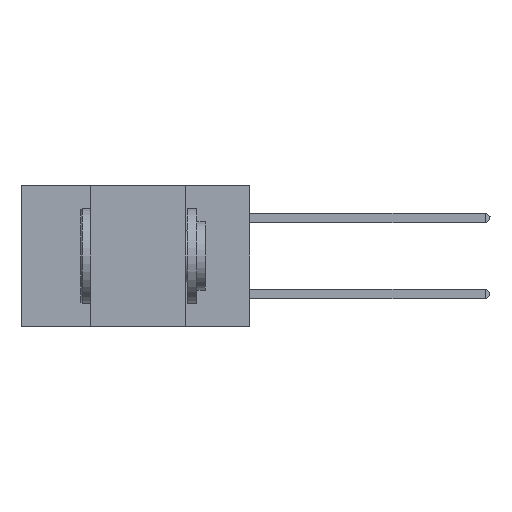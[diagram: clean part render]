
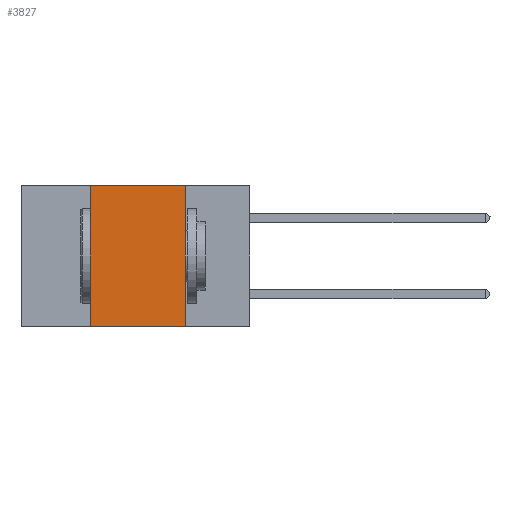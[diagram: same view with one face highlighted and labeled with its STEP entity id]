
A CAD part, left-side view. The second image highlights one B-rep face of the part: STEP entity #3827.
In plain terms, the highlighted planar face has unit normal (-1, 0, 0).
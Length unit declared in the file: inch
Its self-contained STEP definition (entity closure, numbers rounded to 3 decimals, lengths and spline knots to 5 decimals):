
#99 = DIRECTION ( 'NONE',  ( 0., -1., 0. ) ) ;
#1807 = DIRECTION ( 'NONE',  ( 0., -1., 0. ) ) ;
#2031 = VERTEX_POINT ( 'NONE', #17449 ) ;
#2981 = PLANE ( 'NONE',  #18802 ) ;
#3025 = DIRECTION ( 'NONE',  ( 1., 0., 0. ) ) ;
#3157 = CARTESIAN_POINT ( 'NONE',  ( 0., 0.6, 0. ) ) ;
#3827 = ADVANCED_FACE ( 'NONE', ( #16293 ), #2981, .F. ) ;
#4153 = DIRECTION ( 'NONE',  ( 0., 0., 1. ) ) ;
#4222 = LINE ( 'NONE', #20063, #11825 ) ;
#4709 = VECTOR ( 'NONE', #1807, 39.37008 ) ;
#5449 = LINE ( 'NONE', #11422, #9233 ) ;
#5884 = CARTESIAN_POINT ( 'NONE',  ( 0., 0.17, 0. ) ) ;
#6348 = VERTEX_POINT ( 'NONE', #10929 ) ;
#8109 = VERTEX_POINT ( 'NONE', #15239 ) ;
#8470 = EDGE_CURVE ( 'NONE', #9342, #6348, #4222, .T. ) ;
#8858 = ORIENTED_EDGE ( 'NONE', *, *, #19721, .T. ) ;
#8993 = LINE ( 'NONE', #13177, #4709 ) ;
#9233 = VECTOR ( 'NONE', #99, 39.37008 ) ;
#9342 = VERTEX_POINT ( 'NONE', #12723 ) ;
#9894 = EDGE_CURVE ( 'NONE', #2031, #8109, #12808, .T. ) ;
#10929 = CARTESIAN_POINT ( 'NONE',  ( 0., 0.42, 0. ) ) ;
#11422 = CARTESIAN_POINT ( 'NONE',  ( 0., 0.6, -0.37 ) ) ;
#11677 = ORIENTED_EDGE ( 'NONE', *, *, #9894, .F. ) ;
#11825 = VECTOR ( 'NONE', #4153, 39.37008 ) ;
#12196 = ORIENTED_EDGE ( 'NONE', *, *, #18449, .F. ) ;
#12723 = CARTESIAN_POINT ( 'NONE',  ( 0., 0.42, -0.37 ) ) ;
#12808 = LINE ( 'NONE', #5884, #20623 ) ;
#13177 = CARTESIAN_POINT ( 'NONE',  ( 0., 0.6, 0. ) ) ;
#13890 = DIRECTION ( 'NONE',  ( 0., 0., -1. ) ) ;
#14723 = EDGE_LOOP ( 'NONE', ( #11677, #12196, #16944, #8858 ) ) ;
#15239 = CARTESIAN_POINT ( 'NONE',  ( 0., 0.17, -0.37 ) ) ;
#16293 = FACE_OUTER_BOUND ( 'NONE', #14723, .T. ) ;
#16944 = ORIENTED_EDGE ( 'NONE', *, *, #8470, .F. ) ;
#17449 = CARTESIAN_POINT ( 'NONE',  ( 0., 0.17, 0. ) ) ;
#18449 = EDGE_CURVE ( 'NONE', #6348, #2031, #8993, .T. ) ;
#18802 = AXIS2_PLACEMENT_3D ( 'NONE', #3157, #3025, #20419 ) ;
#19721 = EDGE_CURVE ( 'NONE', #9342, #8109, #5449, .T. ) ;
#20063 = CARTESIAN_POINT ( 'NONE',  ( 0., 0.42, 0. ) ) ;
#20419 = DIRECTION ( 'NONE',  ( 0., 0., -1. ) ) ;
#20623 = VECTOR ( 'NONE', #13890, 39.37008 ) ;
